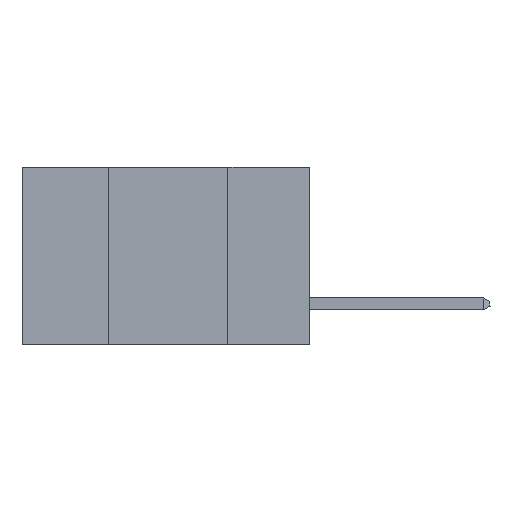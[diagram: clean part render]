
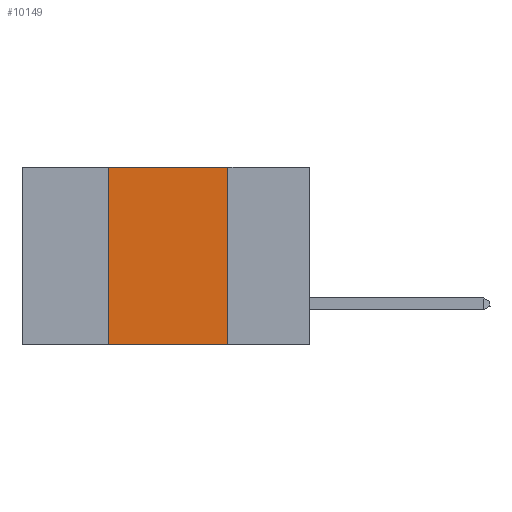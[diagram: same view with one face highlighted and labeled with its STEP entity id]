
A CAD part, left-side view. The second image highlights one B-rep face of the part: STEP entity #10149.
In plain terms, the highlighted planar face has unit normal (-1, 0, 0).
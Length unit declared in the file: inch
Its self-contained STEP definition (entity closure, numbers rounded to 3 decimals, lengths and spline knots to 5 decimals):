
#226 = DIRECTION ( 'NONE',  ( 0., 0., -1. ) ) ;
#501 = LINE ( 'NONE', #15418, #11967 ) ;
#925 = ORIENTED_EDGE ( 'NONE', *, *, #2007, .F. ) ;
#2007 = EDGE_CURVE ( 'NONE', #18012, #19752, #3189, .T. ) ;
#2413 = CARTESIAN_POINT ( 'NONE',  ( 0., 0.42, 0. ) ) ;
#3189 = LINE ( 'NONE', #21406, #14522 ) ;
#5052 = CARTESIAN_POINT ( 'NONE',  ( 0., 0.17, 0. ) ) ;
#6138 = DIRECTION ( 'NONE',  ( 0., 0., 1. ) ) ;
#6368 = DIRECTION ( 'NONE',  ( 0., -1., 0. ) ) ;
#6625 = VERTEX_POINT ( 'NONE', #17769 ) ;
#7903 = ORIENTED_EDGE ( 'NONE', *, *, #19810, .F. ) ;
#8142 = VERTEX_POINT ( 'NONE', #10318 ) ;
#8533 = VECTOR ( 'NONE', #226, 39.37008 ) ;
#8816 = EDGE_LOOP ( 'NONE', ( #7903, #925, #20752, #13053 ) ) ;
#9006 = PLANE ( 'NONE',  #10951 ) ;
#9033 = EDGE_CURVE ( 'NONE', #6625, #18012, #12372, .T. ) ;
#10149 = ADVANCED_FACE ( 'NONE', ( #12060 ), #9006, .F. ) ;
#10318 = CARTESIAN_POINT ( 'NONE',  ( 0., 0.17, -0.37 ) ) ;
#10951 = AXIS2_PLACEMENT_3D ( 'NONE', #18785, #15689, #13604 ) ;
#11967 = VECTOR ( 'NONE', #18724, 39.37008 ) ;
#12060 = FACE_OUTER_BOUND ( 'NONE', #8816, .T. ) ;
#12372 = LINE ( 'NONE', #2413, #20966 ) ;
#12632 = EDGE_CURVE ( 'NONE', #6625, #8142, #501, .T. ) ;
#13053 = ORIENTED_EDGE ( 'NONE', *, *, #12632, .T. ) ;
#13287 = CARTESIAN_POINT ( 'NONE',  ( 0., 0.42, 0. ) ) ;
#13478 = LINE ( 'NONE', #20195, #8533 ) ;
#13604 = DIRECTION ( 'NONE',  ( 0., 0., -1. ) ) ;
#14522 = VECTOR ( 'NONE', #6368, 39.37008 ) ;
#15418 = CARTESIAN_POINT ( 'NONE',  ( 0., 0.6, -0.37 ) ) ;
#15689 = DIRECTION ( 'NONE',  ( 1., 0., 0. ) ) ;
#17769 = CARTESIAN_POINT ( 'NONE',  ( 0., 0.42, -0.37 ) ) ;
#18012 = VERTEX_POINT ( 'NONE', #13287 ) ;
#18724 = DIRECTION ( 'NONE',  ( 0., -1., 0. ) ) ;
#18785 = CARTESIAN_POINT ( 'NONE',  ( 0., 0.6, 0. ) ) ;
#19752 = VERTEX_POINT ( 'NONE', #5052 ) ;
#19810 = EDGE_CURVE ( 'NONE', #19752, #8142, #13478, .T. ) ;
#20195 = CARTESIAN_POINT ( 'NONE',  ( 0., 0.17, 0. ) ) ;
#20752 = ORIENTED_EDGE ( 'NONE', *, *, #9033, .F. ) ;
#20966 = VECTOR ( 'NONE', #6138, 39.37008 ) ;
#21406 = CARTESIAN_POINT ( 'NONE',  ( 0., 0.6, 0. ) ) ;
